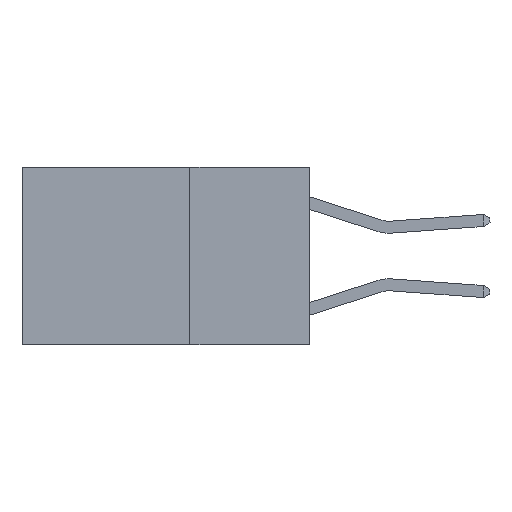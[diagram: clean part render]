
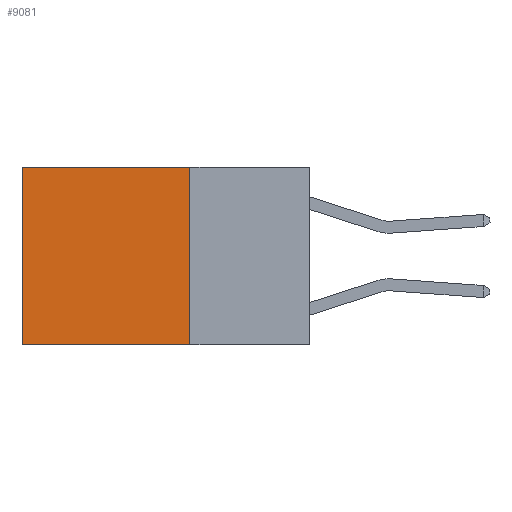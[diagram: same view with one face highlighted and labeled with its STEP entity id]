
A CAD part, left-side view. The second image highlights one B-rep face of the part: STEP entity #9081.
In plain terms, the highlighted planar face has unit normal (-1, 0, 0).
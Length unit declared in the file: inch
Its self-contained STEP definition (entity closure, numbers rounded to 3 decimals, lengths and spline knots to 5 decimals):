
#100 = DIRECTION ( 'NONE',  ( 1., 0., 0. ) ) ;
#103 = LINE ( 'NONE', #3498, #7928 ) ;
#367 = CARTESIAN_POINT ( 'NONE',  ( 0.2625, 0.25, -0.37 ) ) ;
#482 = EDGE_LOOP ( 'NONE', ( #1063, #10633, #6347, #9431 ) ) ;
#574 = EDGE_CURVE ( 'NONE', #5185, #8686, #3122, .T. ) ;
#787 = CARTESIAN_POINT ( 'NONE',  ( 0.2625, 0.6, -0.37 ) ) ;
#851 = VECTOR ( 'NONE', #7286, 39.37008 ) ;
#875 = DIRECTION ( 'NONE',  ( 0., 1., 0. ) ) ;
#1063 = ORIENTED_EDGE ( 'NONE', *, *, #9723, .T. ) ;
#1374 = CARTESIAN_POINT ( 'NONE',  ( 0.2625, 0.6, 0. ) ) ;
#1443 = CARTESIAN_POINT ( 'NONE',  ( 0.2625, 0.25, 0. ) ) ;
#1488 = CARTESIAN_POINT ( 'NONE',  ( 0.2625, 0.25, 0. ) ) ;
#2596 = CARTESIAN_POINT ( 'NONE',  ( 0.2625, 0.25, -0.37 ) ) ;
#3122 = LINE ( 'NONE', #5515, #851 ) ;
#3498 = CARTESIAN_POINT ( 'NONE',  ( 0.2625, 0.6, 0. ) ) ;
#4278 = PLANE ( 'NONE',  #8268 ) ;
#4730 = EDGE_CURVE ( 'NONE', #5185, #5650, #8327, .T. ) ;
#4867 = DIRECTION ( 'NONE',  ( 0., 1., 0. ) ) ;
#5048 = DIRECTION ( 'NONE',  ( 0., 0., -1. ) ) ;
#5185 = VERTEX_POINT ( 'NONE', #1488 ) ;
#5199 = CARTESIAN_POINT ( 'NONE',  ( 0.2625, 0.25, 0. ) ) ;
#5515 = CARTESIAN_POINT ( 'NONE',  ( 0.2625, 0.25, 0. ) ) ;
#5650 = VERTEX_POINT ( 'NONE', #1374 ) ;
#5926 = LINE ( 'NONE', #2596, #6719 ) ;
#5959 = DIRECTION ( 'NONE',  ( 0., 0., -1. ) ) ;
#6347 = ORIENTED_EDGE ( 'NONE', *, *, #574, .F. ) ;
#6719 = VECTOR ( 'NONE', #875, 39.37008 ) ;
#7286 = DIRECTION ( 'NONE',  ( 0., 0., -1. ) ) ;
#7928 = VECTOR ( 'NONE', #5048, 39.37008 ) ;
#8268 = AXIS2_PLACEMENT_3D ( 'NONE', #5199, #100, #5959 ) ;
#8327 = LINE ( 'NONE', #1443, #10023 ) ;
#8488 = FACE_OUTER_BOUND ( 'NONE', #482, .T. ) ;
#8686 = VERTEX_POINT ( 'NONE', #367 ) ;
#9081 = ADVANCED_FACE ( 'NONE', ( #8488 ), #4278, .F. ) ;
#9431 = ORIENTED_EDGE ( 'NONE', *, *, #4730, .T. ) ;
#9545 = VERTEX_POINT ( 'NONE', #787 ) ;
#9723 = EDGE_CURVE ( 'NONE', #5650, #9545, #103, .T. ) ;
#10023 = VECTOR ( 'NONE', #4867, 39.37008 ) ;
#10255 = EDGE_CURVE ( 'NONE', #8686, #9545, #5926, .T. ) ;
#10633 = ORIENTED_EDGE ( 'NONE', *, *, #10255, .F. ) ;
